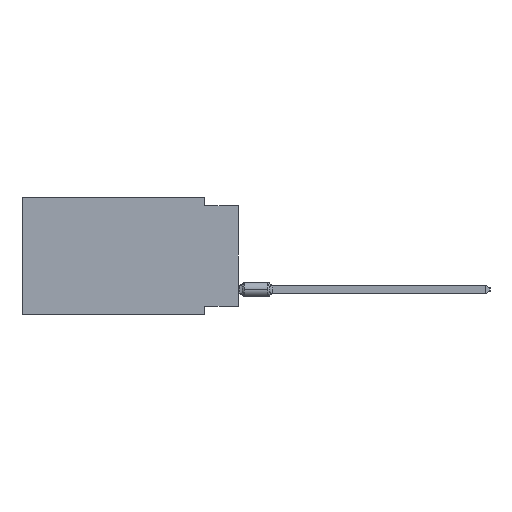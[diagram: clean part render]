
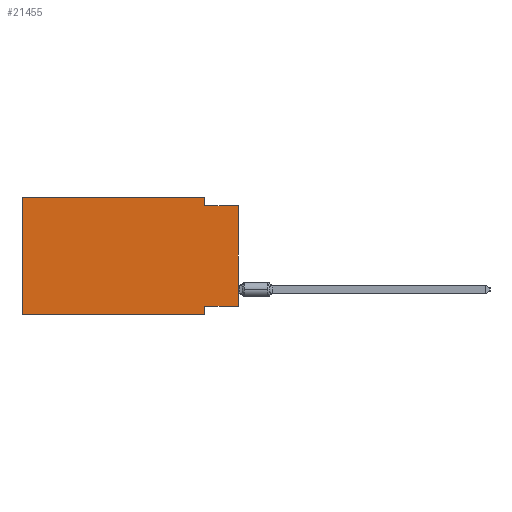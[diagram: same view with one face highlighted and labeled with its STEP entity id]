
A CAD part, left-side view. The second image highlights one B-rep face of the part: STEP entity #21455.
In plain terms, the highlighted planar face has unit normal (-1, 0, 0).
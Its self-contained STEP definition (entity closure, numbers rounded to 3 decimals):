
#542 = VERTEX_POINT ( 'NONE', #53450 ) ;
#898 = VECTOR ( 'NONE', #60072, 1000. ) ;
#1721 = DIRECTION ( 'NONE',  ( 0., 0., 1. ) ) ;
#2160 = EDGE_CURVE ( 'NONE', #18627, #74187, #40367, .T. ) ;
#3157 = VECTOR ( 'NONE', #79134, 1000. ) ;
#4821 = DIRECTION ( 'NONE',  ( 1., 0., 0. ) ) ;
#5644 = DIRECTION ( 'NONE',  ( 0., 0., 1. ) ) ;
#8577 = VECTOR ( 'NONE', #59998, 1000. ) ;
#14696 = ORIENTED_EDGE ( 'NONE', *, *, #80597, .F. ) ;
#15168 = CARTESIAN_POINT ( 'NONE',  ( 0., 0., -8.255 ) ) ;
#17395 = FACE_OUTER_BOUND ( 'NONE', #74210, .T. ) ;
#17574 = CARTESIAN_POINT ( 'NONE',  ( 0., 2.54, -8.255 ) ) ;
#17704 = CARTESIAN_POINT ( 'NONE',  ( 0., 2.54, -8.89 ) ) ;
#18627 = VERTEX_POINT ( 'NONE', #43636 ) ;
#18857 = EDGE_CURVE ( 'NONE', #56220, #61489, #53531, .T. ) ;
#20209 = CARTESIAN_POINT ( 'NONE',  ( 0., 16.383, 0. ) ) ;
#21420 = EDGE_CURVE ( 'NONE', #18627, #61489, #43834, .T. ) ;
#21455 = ADVANCED_FACE ( 'NONE', ( #17395 ), #42987, .F. ) ;
#23411 = VERTEX_POINT ( 'NONE', #24100 ) ;
#24100 = CARTESIAN_POINT ( 'NONE',  ( 0., 2.54, -8.89 ) ) ;
#26308 = ORIENTED_EDGE ( 'NONE', *, *, #39047, .F. ) ;
#28390 = EDGE_CURVE ( 'NONE', #74187, #23411, #50005, .T. ) ;
#30486 = VECTOR ( 'NONE', #5644, 1000. ) ;
#30589 = ORIENTED_EDGE ( 'NONE', *, *, #28390, .F. ) ;
#31111 = DIRECTION ( 'NONE',  ( 0., -1., 0. ) ) ;
#32014 = LINE ( 'NONE', #20209, #75376 ) ;
#34436 = CARTESIAN_POINT ( 'NONE',  ( 0., 16.383, -8.89 ) ) ;
#38095 = ORIENTED_EDGE ( 'NONE', *, *, #44757, .T. ) ;
#38130 = VECTOR ( 'NONE', #31111, 1000. ) ;
#39047 = EDGE_CURVE ( 'NONE', #68711, #542, #63389, .T. ) ;
#40367 = LINE ( 'NONE', #15168, #898 ) ;
#40714 = LINE ( 'NONE', #34436, #8577 ) ;
#42987 = PLANE ( 'NONE',  #53286 ) ;
#43636 = CARTESIAN_POINT ( 'NONE',  ( 0., 0., -8.255 ) ) ;
#43834 = LINE ( 'NONE', #75294, #30486 ) ;
#44008 = CARTESIAN_POINT ( 'NONE',  ( 0., 2.54, -0.635 ) ) ;
#44165 = VERTEX_POINT ( 'NONE', #61525 ) ;
#44455 = CARTESIAN_POINT ( 'NONE',  ( 0., 0., -0.635 ) ) ;
#44757 = EDGE_CURVE ( 'NONE', #44165, #23411, #40714, .T. ) ;
#45057 = DIRECTION ( 'NONE',  ( 0., 0., -1. ) ) ;
#45889 = CARTESIAN_POINT ( 'NONE',  ( 0., 16.383, 0. ) ) ;
#48070 = VECTOR ( 'NONE', #49737, 1000. ) ;
#49737 = DIRECTION ( 'NONE',  ( 0., 0., -1. ) ) ;
#50005 = LINE ( 'NONE', #17704, #67302 ) ;
#53286 = AXIS2_PLACEMENT_3D ( 'NONE', #62281, #4821, #45057 ) ;
#53450 = CARTESIAN_POINT ( 'NONE',  ( 0., 2.54, 0. ) ) ;
#53531 = LINE ( 'NONE', #44455, #3157 ) ;
#54585 = ORIENTED_EDGE ( 'NONE', *, *, #18857, .F. ) ;
#56220 = VERTEX_POINT ( 'NONE', #44008 ) ;
#57119 = CARTESIAN_POINT ( 'NONE',  ( 0., 16.383, 0. ) ) ;
#59998 = DIRECTION ( 'NONE',  ( 0., -1., 0. ) ) ;
#60072 = DIRECTION ( 'NONE',  ( 0., 1., 0. ) ) ;
#60660 = CARTESIAN_POINT ( 'NONE',  ( 0., 2.54, 0. ) ) ;
#61489 = VERTEX_POINT ( 'NONE', #80764 ) ;
#61525 = CARTESIAN_POINT ( 'NONE',  ( 0., 16.383, -8.89 ) ) ;
#62281 = CARTESIAN_POINT ( 'NONE',  ( 0., 16.383, 0. ) ) ;
#63389 = LINE ( 'NONE', #57119, #38130 ) ;
#63582 = EDGE_CURVE ( 'NONE', #542, #56220, #74523, .T. ) ;
#67302 = VECTOR ( 'NONE', #69722, 1000. ) ;
#68711 = VERTEX_POINT ( 'NONE', #45889 ) ;
#69722 = DIRECTION ( 'NONE',  ( 0., 0., -1. ) ) ;
#74187 = VERTEX_POINT ( 'NONE', #17574 ) ;
#74210 = EDGE_LOOP ( 'NONE', ( #76063, #54585, #81737, #26308, #14696, #38095, #30589, #81721 ) ) ;
#74523 = LINE ( 'NONE', #60660, #48070 ) ;
#75294 = CARTESIAN_POINT ( 'NONE',  ( 0., 0., 0. ) ) ;
#75376 = VECTOR ( 'NONE', #1721, 1000. ) ;
#76063 = ORIENTED_EDGE ( 'NONE', *, *, #21420, .T. ) ;
#79134 = DIRECTION ( 'NONE',  ( 0., -1., 0. ) ) ;
#80597 = EDGE_CURVE ( 'NONE', #44165, #68711, #32014, .T. ) ;
#80764 = CARTESIAN_POINT ( 'NONE',  ( 0., 0., -0.635 ) ) ;
#81721 = ORIENTED_EDGE ( 'NONE', *, *, #2160, .F. ) ;
#81737 = ORIENTED_EDGE ( 'NONE', *, *, #63582, .F. ) ;
